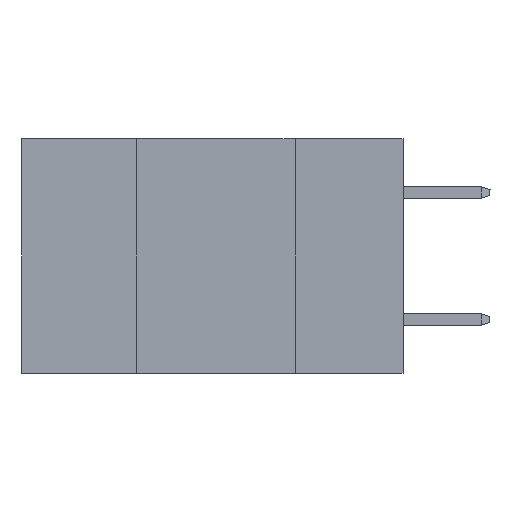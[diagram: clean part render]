
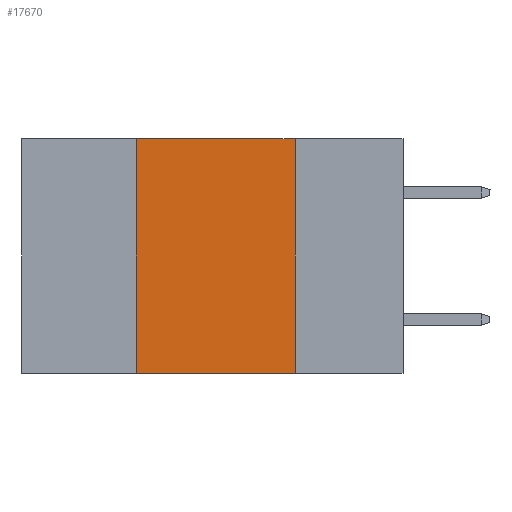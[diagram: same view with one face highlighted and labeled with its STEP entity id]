
A CAD part, left-side view. The second image highlights one B-rep face of the part: STEP entity #17670.
In plain terms, the highlighted planar face has unit normal (-1, 0, 0).
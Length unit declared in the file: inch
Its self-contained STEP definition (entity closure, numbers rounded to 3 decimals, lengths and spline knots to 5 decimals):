
#205 = DIRECTION ( 'NONE',  ( 0., -1., 0. ) ) ;
#231 = CARTESIAN_POINT ( 'NONE',  ( 0., 0.17, 0. ) ) ;
#369 = VERTEX_POINT ( 'NONE', #8811 ) ;
#1634 = PLANE ( 'NONE',  #20176 ) ;
#2151 = VERTEX_POINT ( 'NONE', #231 ) ;
#2216 = EDGE_CURVE ( 'NONE', #19174, #4653, #20349, .T. ) ;
#2658 = ORIENTED_EDGE ( 'NONE', *, *, #2708, .F. ) ;
#2708 = EDGE_CURVE ( 'NONE', #4653, #2151, #10161, .T. ) ;
#3270 = FACE_OUTER_BOUND ( 'NONE', #14576, .T. ) ;
#3624 = DIRECTION ( 'NONE',  ( 0., -1., 0. ) ) ;
#3783 = VECTOR ( 'NONE', #21175, 39.37008 ) ;
#4653 = VERTEX_POINT ( 'NONE', #7871 ) ;
#4744 = CARTESIAN_POINT ( 'NONE',  ( 0., 0.17, 0. ) ) ;
#5233 = CARTESIAN_POINT ( 'NONE',  ( 0., 0.42, -0.37 ) ) ;
#5449 = DIRECTION ( 'NONE',  ( 0., 0., 1. ) ) ;
#5458 = ORIENTED_EDGE ( 'NONE', *, *, #18258, .T. ) ;
#6891 = CARTESIAN_POINT ( 'NONE',  ( 0., 0.6, 0. ) ) ;
#7506 = ORIENTED_EDGE ( 'NONE', *, *, #9416, .F. ) ;
#7871 = CARTESIAN_POINT ( 'NONE',  ( 0., 0.42, 0. ) ) ;
#8811 = CARTESIAN_POINT ( 'NONE',  ( 0., 0.17, -0.37 ) ) ;
#9416 = EDGE_CURVE ( 'NONE', #2151, #369, #9495, .T. ) ;
#9495 = LINE ( 'NONE', #4744, #3783 ) ;
#10161 = LINE ( 'NONE', #15167, #15521 ) ;
#10241 = LINE ( 'NONE', #10561, #18838 ) ;
#10561 = CARTESIAN_POINT ( 'NONE',  ( 0., 0.6, -0.37 ) ) ;
#13563 = DIRECTION ( 'NONE',  ( 1., 0., 0. ) ) ;
#13803 = VECTOR ( 'NONE', #5449, 39.37008 ) ;
#14576 = EDGE_LOOP ( 'NONE', ( #7506, #2658, #20780, #5458 ) ) ;
#15167 = CARTESIAN_POINT ( 'NONE',  ( 0., 0.6, 0. ) ) ;
#15516 = CARTESIAN_POINT ( 'NONE',  ( 0., 0.42, 0. ) ) ;
#15521 = VECTOR ( 'NONE', #205, 39.37008 ) ;
#17670 = ADVANCED_FACE ( 'NONE', ( #3270 ), #1634, .F. ) ;
#18258 = EDGE_CURVE ( 'NONE', #19174, #369, #10241, .T. ) ;
#18838 = VECTOR ( 'NONE', #3624, 39.37008 ) ;
#19174 = VERTEX_POINT ( 'NONE', #5233 ) ;
#20155 = DIRECTION ( 'NONE',  ( 0., 0., -1. ) ) ;
#20176 = AXIS2_PLACEMENT_3D ( 'NONE', #6891, #13563, #20155 ) ;
#20349 = LINE ( 'NONE', #15516, #13803 ) ;
#20780 = ORIENTED_EDGE ( 'NONE', *, *, #2216, .F. ) ;
#21175 = DIRECTION ( 'NONE',  ( 0., 0., -1. ) ) ;
